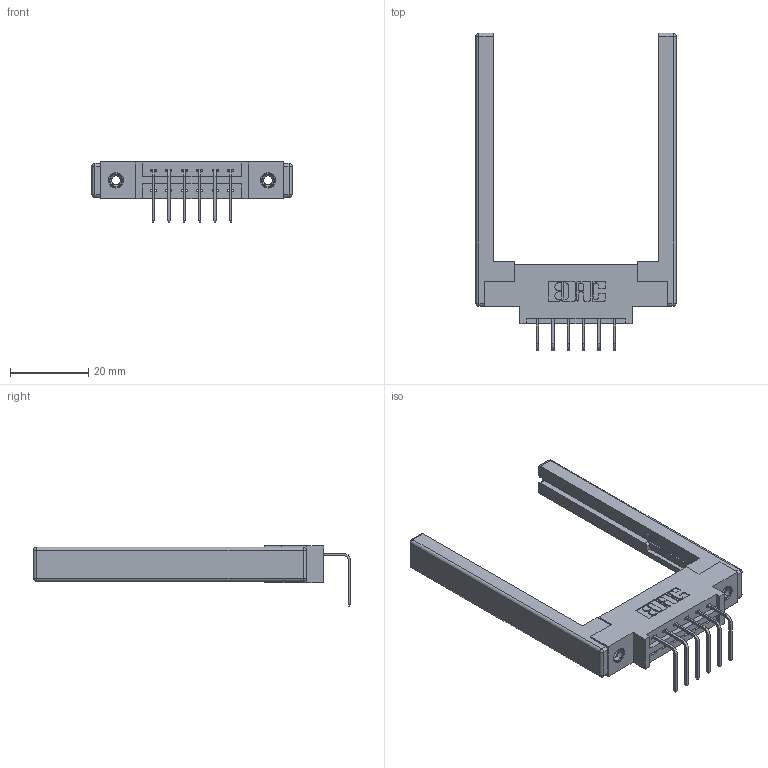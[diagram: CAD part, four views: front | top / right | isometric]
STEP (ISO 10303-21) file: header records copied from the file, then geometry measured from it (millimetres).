
FILE_DESCRIPTION (( 'STEP AP203' ), '1' );
FILE_NAME ('387-006-558-668.STEP', '2019-10-07T15:45:06', ( '' ), ( '' ), 'SwSTEP 2.0', 'SolidWorks 2016', '' );
FILE_SCHEMA (( 'CONFIG_CONTROL_DESIGN' ));
Length unit declared in the file: inch
Products named in the file (5): 345-250-001_345-250-001-102; 345-292-001_558 Tail - 2; 337 Part_0.170 Offset - 0.156 Dia-TI; 387-006-558-668; 307-220-068
Assembly tree (11 placements, depth 2):
  387-006-558-668
    337 Part_0.170 Offset - 0.156 Dia-TI
    345-292-001_558 Tail - 2  x6
    345-250-001_345-250-001-102  x2
    307-220-068  x2
Bounding box: 51.21 x 81.22 x 15.37 mm (x, y, z)
Volume: 9165.3 mm3; surface area: 9045.4 mm2
Topology: 11 solids, 11 shells, 656 faces, 1877 edges, 1222 vertices
Faces by surface type: plane 450, cylinder 182, cone 12, sphere 8, torus 4
Entity records: 12092 total; most frequent: CARTESIAN_POINT 2061, ORIENTED_EDGE 1992, DIRECTION 1882, EDGE_CURVE 996, LINE 818, VECTOR 818, VERTEX_POINT 654, AXIS2_PLACEMENT_3D 532
